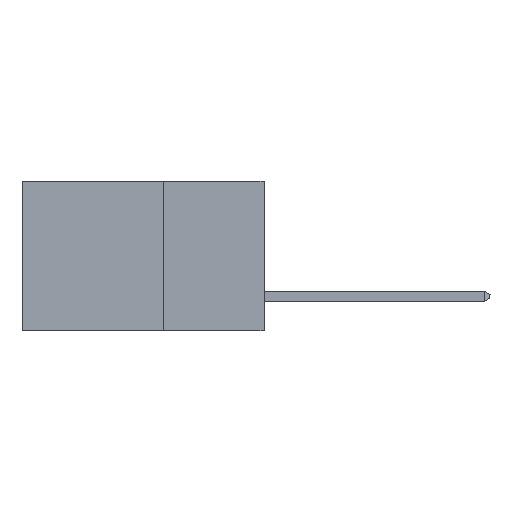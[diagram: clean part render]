
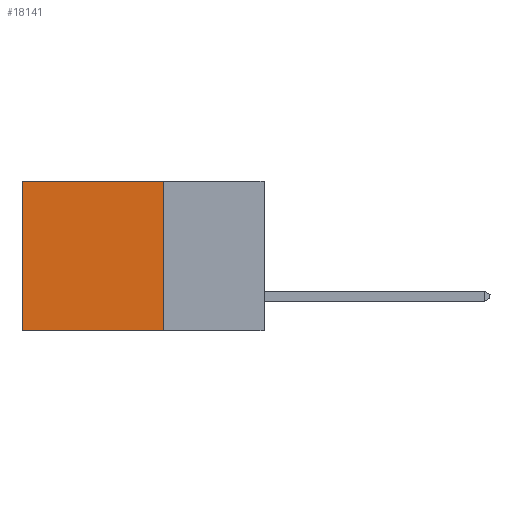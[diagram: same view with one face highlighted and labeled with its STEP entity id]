
A CAD part, left-side view. The second image highlights one B-rep face of the part: STEP entity #18141.
In plain terms, the highlighted planar face has unit normal (-1, 0, 0).
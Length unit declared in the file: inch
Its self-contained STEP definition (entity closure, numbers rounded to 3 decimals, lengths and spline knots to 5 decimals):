
#1078 = CARTESIAN_POINT ( 'NONE',  ( 0.298, 0.25, 0. ) ) ;
#2247 = VERTEX_POINT ( 'NONE', #5826 ) ;
#2684 = EDGE_CURVE ( 'NONE', #15871, #2247, #26806, .T. ) ;
#2733 = VERTEX_POINT ( 'NONE', #19498 ) ;
#3851 = CARTESIAN_POINT ( 'NONE',  ( 0.298, 0.25, 0. ) ) ;
#4062 = CARTESIAN_POINT ( 'NONE',  ( 0.298, 0.6, 0. ) ) ;
#4467 = EDGE_LOOP ( 'NONE', ( #27268, #15606, #4649, #6450 ) ) ;
#4649 = ORIENTED_EDGE ( 'NONE', *, *, #16499, .F. ) ;
#5251 = VERTEX_POINT ( 'NONE', #19528 ) ;
#5826 = CARTESIAN_POINT ( 'NONE',  ( 0.298, 0.6, -0.37 ) ) ;
#6450 = ORIENTED_EDGE ( 'NONE', *, *, #18063, .T. ) ;
#9273 = VECTOR ( 'NONE', #12686, 39.37008 ) ;
#12118 = CARTESIAN_POINT ( 'NONE',  ( 0.298, 0.25, 0. ) ) ;
#12686 = DIRECTION ( 'NONE',  ( 0., 1., 0. ) ) ;
#13590 = AXIS2_PLACEMENT_3D ( 'NONE', #3851, #19287, #15111 ) ;
#14100 = VECTOR ( 'NONE', #20784, 39.37008 ) ;
#15111 = DIRECTION ( 'NONE',  ( 0., 0., -1. ) ) ;
#15606 = ORIENTED_EDGE ( 'NONE', *, *, #18550, .F. ) ;
#15871 = VERTEX_POINT ( 'NONE', #16406 ) ;
#16151 = CARTESIAN_POINT ( 'NONE',  ( 0.298, 0.25, -0.37 ) ) ;
#16180 = LINE ( 'NONE', #16151, #14100 ) ;
#16406 = CARTESIAN_POINT ( 'NONE',  ( 0.298, 0.6, 0. ) ) ;
#16499 = EDGE_CURVE ( 'NONE', #5251, #2733, #23220, .T. ) ;
#16659 = VECTOR ( 'NONE', #23491, 39.37008 ) ;
#16746 = VECTOR ( 'NONE', #26370, 39.37008 ) ;
#18063 = EDGE_CURVE ( 'NONE', #5251, #15871, #22789, .T. ) ;
#18141 = ADVANCED_FACE ( 'NONE', ( #22107 ), #26138, .F. ) ;
#18550 = EDGE_CURVE ( 'NONE', #2733, #2247, #16180, .T. ) ;
#19287 = DIRECTION ( 'NONE',  ( 1., 0., 0. ) ) ;
#19498 = CARTESIAN_POINT ( 'NONE',  ( 0.298, 0.25, -0.37 ) ) ;
#19528 = CARTESIAN_POINT ( 'NONE',  ( 0.298, 0.25, 0. ) ) ;
#20784 = DIRECTION ( 'NONE',  ( 0., 1., 0. ) ) ;
#22107 = FACE_OUTER_BOUND ( 'NONE', #4467, .T. ) ;
#22789 = LINE ( 'NONE', #12118, #9273 ) ;
#23220 = LINE ( 'NONE', #1078, #16659 ) ;
#23491 = DIRECTION ( 'NONE',  ( 0., 0., -1. ) ) ;
#26138 = PLANE ( 'NONE',  #13590 ) ;
#26370 = DIRECTION ( 'NONE',  ( 0., 0., -1. ) ) ;
#26806 = LINE ( 'NONE', #4062, #16746 ) ;
#27268 = ORIENTED_EDGE ( 'NONE', *, *, #2684, .T. ) ;
